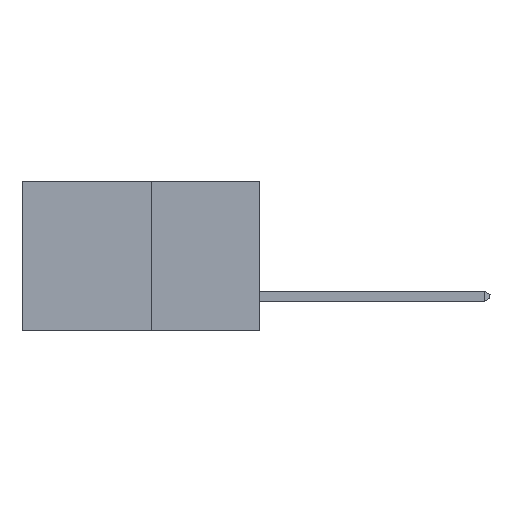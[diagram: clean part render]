
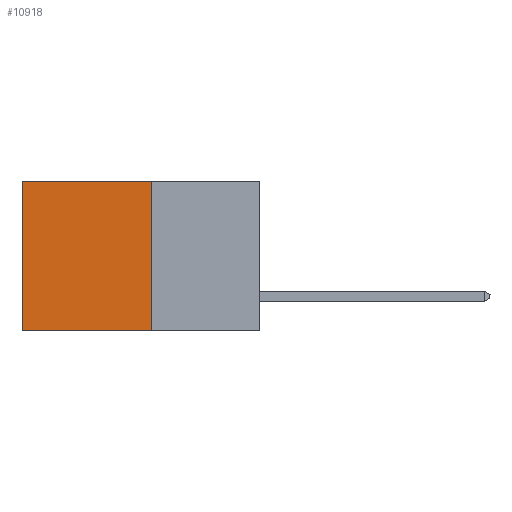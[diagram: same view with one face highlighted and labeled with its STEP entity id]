
A CAD part, left-side view. The second image highlights one B-rep face of the part: STEP entity #10918.
In plain terms, the highlighted planar face has unit normal (-1, 0, 0).
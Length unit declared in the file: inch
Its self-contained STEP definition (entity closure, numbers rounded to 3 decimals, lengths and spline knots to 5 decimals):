
#327 = CARTESIAN_POINT ( 'NONE',  ( 0.277, 0.27, -0.37 ) ) ;
#520 = CARTESIAN_POINT ( 'NONE',  ( 0.277, 0.27, -0.37 ) ) ;
#566 = CARTESIAN_POINT ( 'NONE',  ( 0.277, 0.59, 0. ) ) ;
#736 = EDGE_CURVE ( 'NONE', #6770, #5304, #11657, .T. ) ;
#939 = EDGE_LOOP ( 'NONE', ( #1093, #5555, #9251, #13512 ) ) ;
#1093 = ORIENTED_EDGE ( 'NONE', *, *, #3700, .T. ) ;
#1704 = PLANE ( 'NONE',  #10161 ) ;
#1801 = CARTESIAN_POINT ( 'NONE',  ( 0.277, 0.59, -0.37 ) ) ;
#2303 = LINE ( 'NONE', #1801, #11138 ) ;
#2581 = EDGE_CURVE ( 'NONE', #9215, #6770, #13912, .T. ) ;
#3642 = FACE_OUTER_BOUND ( 'NONE', #939, .T. ) ;
#3700 = EDGE_CURVE ( 'NONE', #14573, #5304, #2303, .T. ) ;
#4375 = CARTESIAN_POINT ( 'NONE',  ( 0.277, 0.27, 0. ) ) ;
#4618 = DIRECTION ( 'NONE',  ( 0., 1., 0. ) ) ;
#5304 = VERTEX_POINT ( 'NONE', #13351 ) ;
#5555 = ORIENTED_EDGE ( 'NONE', *, *, #736, .F. ) ;
#6770 = VERTEX_POINT ( 'NONE', #14366 ) ;
#6785 = DIRECTION ( 'NONE',  ( 0., 0., -1. ) ) ;
#9215 = VERTEX_POINT ( 'NONE', #12178 ) ;
#9251 = ORIENTED_EDGE ( 'NONE', *, *, #2581, .F. ) ;
#9894 = DIRECTION ( 'NONE',  ( 0., 0., -1. ) ) ;
#10161 = AXIS2_PLACEMENT_3D ( 'NONE', #520, #11972, #9894 ) ;
#10918 = ADVANCED_FACE ( 'NONE', ( #3642 ), #1704, .F. ) ;
#11042 = EDGE_CURVE ( 'NONE', #9215, #14573, #11605, .T. ) ;
#11138 = VECTOR ( 'NONE', #6785, 39.37008 ) ;
#11186 = VECTOR ( 'NONE', #12124, 39.37008 ) ;
#11605 = LINE ( 'NONE', #4375, #11921 ) ;
#11657 = LINE ( 'NONE', #327, #14380 ) ;
#11921 = VECTOR ( 'NONE', #12150, 39.37008 ) ;
#11972 = DIRECTION ( 'NONE',  ( 1., 0., 0. ) ) ;
#12107 = CARTESIAN_POINT ( 'NONE',  ( 0.277, 0.27, -0.37 ) ) ;
#12124 = DIRECTION ( 'NONE',  ( 0., 0., -1. ) ) ;
#12150 = DIRECTION ( 'NONE',  ( 0., 1., 0. ) ) ;
#12178 = CARTESIAN_POINT ( 'NONE',  ( 0.277, 0.27, 0. ) ) ;
#13351 = CARTESIAN_POINT ( 'NONE',  ( 0.277, 0.59, -0.37 ) ) ;
#13512 = ORIENTED_EDGE ( 'NONE', *, *, #11042, .T. ) ;
#13912 = LINE ( 'NONE', #12107, #11186 ) ;
#14366 = CARTESIAN_POINT ( 'NONE',  ( 0.277, 0.27, -0.37 ) ) ;
#14380 = VECTOR ( 'NONE', #4618, 39.37008 ) ;
#14573 = VERTEX_POINT ( 'NONE', #566 ) ;
